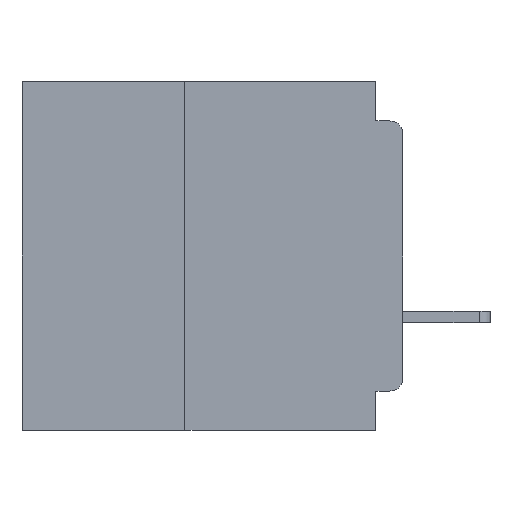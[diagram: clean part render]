
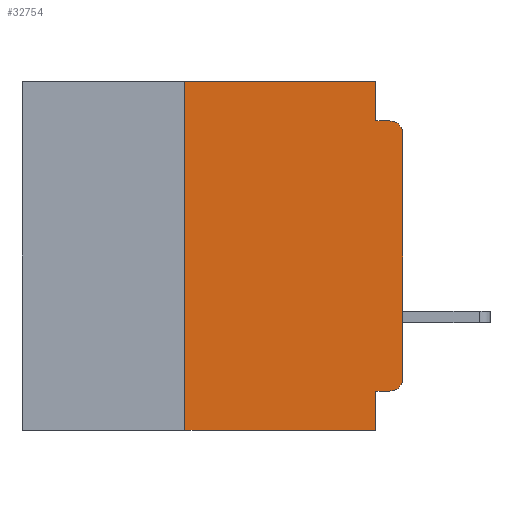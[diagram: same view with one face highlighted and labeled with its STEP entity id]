
A CAD part, left-side view. The second image highlights one B-rep face of the part: STEP entity #32754.
In plain terms, the highlighted planar face has unit normal (-1, 0, 0).
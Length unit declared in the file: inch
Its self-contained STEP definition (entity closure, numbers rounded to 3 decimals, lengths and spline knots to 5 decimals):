
#16 = CARTESIAN_POINT ( 'NONE',  ( 0., 0.031, -0.045 ) ) ;
#706 = CARTESIAN_POINT ( 'NONE',  ( 0., 0.015, -0.045 ) ) ;
#983 = VECTOR ( 'NONE', #54063, 39.37008 ) ;
#1649 = ORIENTED_EDGE ( 'NONE', *, *, #49563, .F. ) ;
#1761 = LINE ( 'NONE', #42323, #34832 ) ;
#5423 = CARTESIAN_POINT ( 'NONE',  ( 0., 0., -0.34 ) ) ;
#6945 = VERTEX_POINT ( 'NONE', #47658 ) ;
#7119 = ORIENTED_EDGE ( 'NONE', *, *, #27341, .F. ) ;
#7411 = EDGE_CURVE ( 'NONE', #44737, #27817, #1761, .T. ) ;
#7570 = CIRCLE ( 'NONE', #32890, 0.015 ) ;
#8272 = LINE ( 'NONE', #20428, #31242 ) ;
#9063 = DIRECTION ( 'NONE',  ( 0., 0., -1. ) ) ;
#9219 = DIRECTION ( 'NONE',  ( 0., -1., 0. ) ) ;
#11233 = FACE_OUTER_BOUND ( 'NONE', #52243, .T. ) ;
#11555 = VERTEX_POINT ( 'NONE', #19285 ) ;
#11709 = DIRECTION ( 'NONE',  ( -1., 0., 0. ) ) ;
#12622 = DIRECTION ( 'NONE',  ( 0., 0., 1. ) ) ;
#12878 = EDGE_CURVE ( 'NONE', #21541, #27817, #17233, .T. ) ;
#13795 = ORIENTED_EDGE ( 'NONE', *, *, #54442, .F. ) ;
#15070 = CARTESIAN_POINT ( 'NONE',  ( 0., 0.437, 0. ) ) ;
#17233 = CIRCLE ( 'NONE', #24428, 0.015 ) ;
#18166 = ORIENTED_EDGE ( 'NONE', *, *, #7411, .F. ) ;
#18255 = DIRECTION ( 'NONE',  ( 0., 0., -1. ) ) ;
#19285 = CARTESIAN_POINT ( 'NONE',  ( 0., 0.031, -0.4 ) ) ;
#19573 = LINE ( 'NONE', #34061, #41020 ) ;
#20428 = CARTESIAN_POINT ( 'NONE',  ( 0., 0., 0. ) ) ;
#20961 = VECTOR ( 'NONE', #29842, 39.37008 ) ;
#21541 = VERTEX_POINT ( 'NONE', #27020 ) ;
#21973 = CARTESIAN_POINT ( 'NONE',  ( 0., 0.437, 0. ) ) ;
#22124 = EDGE_CURVE ( 'NONE', #46909, #11555, #53162, .T. ) ;
#24060 = ORIENTED_EDGE ( 'NONE', *, *, #22124, .T. ) ;
#24100 = LINE ( 'NONE', #45281, #983 ) ;
#24417 = CARTESIAN_POINT ( 'NONE',  ( 0., 0.031, 0. ) ) ;
#24428 = AXIS2_PLACEMENT_3D ( 'NONE', #37475, #11709, #41812 ) ;
#24612 = CARTESIAN_POINT ( 'NONE',  ( 0., 0.015, -0.34 ) ) ;
#25506 = CARTESIAN_POINT ( 'NONE',  ( 0., 0.015, -0.355 ) ) ;
#25545 = CARTESIAN_POINT ( 'NONE',  ( 0., 0., -0.355 ) ) ;
#25944 = ORIENTED_EDGE ( 'NONE', *, *, #29365, .T. ) ;
#27020 = CARTESIAN_POINT ( 'NONE',  ( 0., 0., -0.06 ) ) ;
#27341 = EDGE_CURVE ( 'NONE', #38233, #39469, #35104, .T. ) ;
#27817 = VERTEX_POINT ( 'NONE', #706 ) ;
#28676 = AXIS2_PLACEMENT_3D ( 'NONE', #21973, #34856, #9063 ) ;
#28888 = DIRECTION ( 'NONE',  ( 0., 0., -1. ) ) ;
#29365 = EDGE_CURVE ( 'NONE', #36002, #42080, #7570, .T. ) ;
#29842 = DIRECTION ( 'NONE',  ( 0., 1., 0. ) ) ;
#30308 = VECTOR ( 'NONE', #9219, 39.37008 ) ;
#30568 = PLANE ( 'NONE',  #28676 ) ;
#31000 = CARTESIAN_POINT ( 'NONE',  ( 0., 0.031, -0.4 ) ) ;
#31242 = VECTOR ( 'NONE', #37434, 39.37008 ) ;
#32739 = ORIENTED_EDGE ( 'NONE', *, *, #40896, .F. ) ;
#32754 = ADVANCED_FACE ( 'NONE', ( #11233 ), #30568, .F. ) ;
#32890 = AXIS2_PLACEMENT_3D ( 'NONE', #24612, #54602, #28888 ) ;
#33269 = CARTESIAN_POINT ( 'NONE',  ( 0., 0.25, -0.4 ) ) ;
#33874 = DIRECTION ( 'NONE',  ( 0., -1., 0. ) ) ;
#34061 = CARTESIAN_POINT ( 'NONE',  ( 0., 0.25, -0.4 ) ) ;
#34763 = EDGE_CURVE ( 'NONE', #46909, #38233, #19573, .T. ) ;
#34832 = VECTOR ( 'NONE', #33874, 39.37008 ) ;
#34856 = DIRECTION ( 'NONE',  ( 1., 0., 0. ) ) ;
#35104 = LINE ( 'NONE', #15070, #36460 ) ;
#36002 = VERTEX_POINT ( 'NONE', #25506 ) ;
#36460 = VECTOR ( 'NONE', #45137, 39.37008 ) ;
#37434 = DIRECTION ( 'NONE',  ( 0., 0., 1. ) ) ;
#37475 = CARTESIAN_POINT ( 'NONE',  ( 0., 0.015, -0.06 ) ) ;
#38233 = VERTEX_POINT ( 'NONE', #52262 ) ;
#39312 = CARTESIAN_POINT ( 'NONE',  ( 0., 0.437, -0.4 ) ) ;
#39469 = VERTEX_POINT ( 'NONE', #24417 ) ;
#39821 = ORIENTED_EDGE ( 'NONE', *, *, #12878, .T. ) ;
#40896 = EDGE_CURVE ( 'NONE', #36002, #6945, #43756, .T. ) ;
#41020 = VECTOR ( 'NONE', #12622, 39.37008 ) ;
#41812 = DIRECTION ( 'NONE',  ( 0., 0., -1. ) ) ;
#42080 = VERTEX_POINT ( 'NONE', #5423 ) ;
#42323 = CARTESIAN_POINT ( 'NONE',  ( 0., 0., -0.045 ) ) ;
#43756 = LINE ( 'NONE', #25545, #20961 ) ;
#44737 = VERTEX_POINT ( 'NONE', #16 ) ;
#45137 = DIRECTION ( 'NONE',  ( 0., -1., 0. ) ) ;
#45281 = CARTESIAN_POINT ( 'NONE',  ( 0., 0.031, 0. ) ) ;
#46909 = VERTEX_POINT ( 'NONE', #33269 ) ;
#47658 = CARTESIAN_POINT ( 'NONE',  ( 0., 0.031, -0.355 ) ) ;
#48616 = EDGE_CURVE ( 'NONE', #42080, #21541, #8272, .T. ) ;
#48867 = ORIENTED_EDGE ( 'NONE', *, *, #34763, .F. ) ;
#49524 = ORIENTED_EDGE ( 'NONE', *, *, #48616, .T. ) ;
#49563 = EDGE_CURVE ( 'NONE', #6945, #11555, #51256, .T. ) ;
#49939 = VECTOR ( 'NONE', #18255, 39.37008 ) ;
#51256 = LINE ( 'NONE', #31000, #49939 ) ;
#52243 = EDGE_LOOP ( 'NONE', ( #49524, #39821, #18166, #13795, #7119, #48867, #24060, #1649, #32739, #25944 ) ) ;
#52262 = CARTESIAN_POINT ( 'NONE',  ( 0., 0.25, 0. ) ) ;
#53162 = LINE ( 'NONE', #39312, #30308 ) ;
#54063 = DIRECTION ( 'NONE',  ( 0., 0., -1. ) ) ;
#54442 = EDGE_CURVE ( 'NONE', #39469, #44737, #24100, .T. ) ;
#54602 = DIRECTION ( 'NONE',  ( -1., 0., 0. ) ) ;
